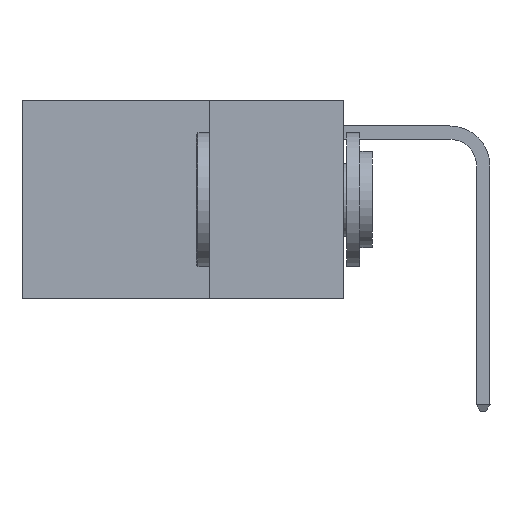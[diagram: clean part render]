
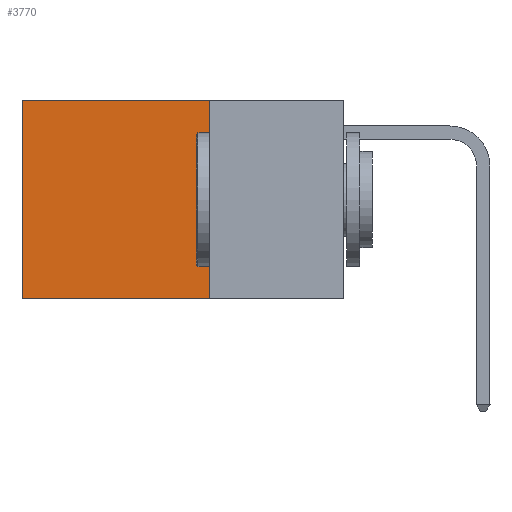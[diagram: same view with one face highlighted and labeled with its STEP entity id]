
A CAD part, left-side view. The second image highlights one B-rep face of the part: STEP entity #3770.
In plain terms, the highlighted planar face has unit normal (-1, 0, 0).
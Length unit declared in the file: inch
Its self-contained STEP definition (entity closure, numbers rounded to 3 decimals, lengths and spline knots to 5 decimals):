
#184 = EDGE_LOOP ( 'NONE', ( #5452, #452, #4690, #10285 ) ) ;
#452 = ORIENTED_EDGE ( 'NONE', *, *, #1931, .F. ) ;
#627 = VECTOR ( 'NONE', #13484, 39.37008 ) ;
#949 = LINE ( 'NONE', #13482, #627 ) ;
#1931 = EDGE_CURVE ( 'NONE', #4894, #4865, #4077, .T. ) ;
#2164 = CARTESIAN_POINT ( 'NONE',  ( 0.2625, 0.25, -0.37 ) ) ;
#2760 = CARTESIAN_POINT ( 'NONE',  ( 0.2625, 0.25, 0. ) ) ;
#3146 = AXIS2_PLACEMENT_3D ( 'NONE', #5284, #5101, #5087 ) ;
#3155 = CARTESIAN_POINT ( 'NONE',  ( 0.2625, 0.6, -0.37 ) ) ;
#3656 = DIRECTION ( 'NONE',  ( 0., 1., 0. ) ) ;
#3770 = ADVANCED_FACE ( 'NONE', ( #13049 ), #5120, .F. ) ;
#4077 = LINE ( 'NONE', #13591, #4235 ) ;
#4235 = VECTOR ( 'NONE', #4921, 39.37008 ) ;
#4690 = ORIENTED_EDGE ( 'NONE', *, *, #7959, .F. ) ;
#4865 = VERTEX_POINT ( 'NONE', #3155 ) ;
#4867 = EDGE_CURVE ( 'NONE', #9717, #13782, #9157, .T. ) ;
#4894 = VERTEX_POINT ( 'NONE', #2164 ) ;
#4921 = DIRECTION ( 'NONE',  ( 0., 1., 0. ) ) ;
#5087 = DIRECTION ( 'NONE',  ( 0., 0., -1. ) ) ;
#5101 = DIRECTION ( 'NONE',  ( 1., 0., 0. ) ) ;
#5120 = PLANE ( 'NONE',  #3146 ) ;
#5284 = CARTESIAN_POINT ( 'NONE',  ( 0.2625, 0.25, 0. ) ) ;
#5452 = ORIENTED_EDGE ( 'NONE', *, *, #7300, .T. ) ;
#5700 = LINE ( 'NONE', #13052, #14097 ) ;
#7300 = EDGE_CURVE ( 'NONE', #13782, #4865, #5700, .T. ) ;
#7959 = EDGE_CURVE ( 'NONE', #9717, #4894, #949, .T. ) ;
#8410 = CARTESIAN_POINT ( 'NONE',  ( 0.2625, 0.25, 0. ) ) ;
#9143 = VECTOR ( 'NONE', #3656, 39.37008 ) ;
#9157 = LINE ( 'NONE', #2760, #9143 ) ;
#9717 = VERTEX_POINT ( 'NONE', #8410 ) ;
#10285 = ORIENTED_EDGE ( 'NONE', *, *, #4867, .T. ) ;
#12057 = CARTESIAN_POINT ( 'NONE',  ( 0.2625, 0.6, 0. ) ) ;
#12972 = DIRECTION ( 'NONE',  ( 0., 0., -1. ) ) ;
#13049 = FACE_OUTER_BOUND ( 'NONE', #184, .T. ) ;
#13052 = CARTESIAN_POINT ( 'NONE',  ( 0.2625, 0.6, 0. ) ) ;
#13482 = CARTESIAN_POINT ( 'NONE',  ( 0.2625, 0.25, 0. ) ) ;
#13484 = DIRECTION ( 'NONE',  ( 0., 0., -1. ) ) ;
#13591 = CARTESIAN_POINT ( 'NONE',  ( 0.2625, 0.25, -0.37 ) ) ;
#13782 = VERTEX_POINT ( 'NONE', #12057 ) ;
#14097 = VECTOR ( 'NONE', #12972, 39.37008 ) ;
